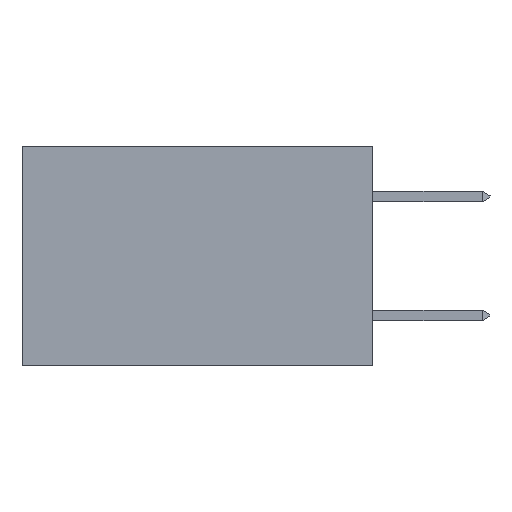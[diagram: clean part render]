
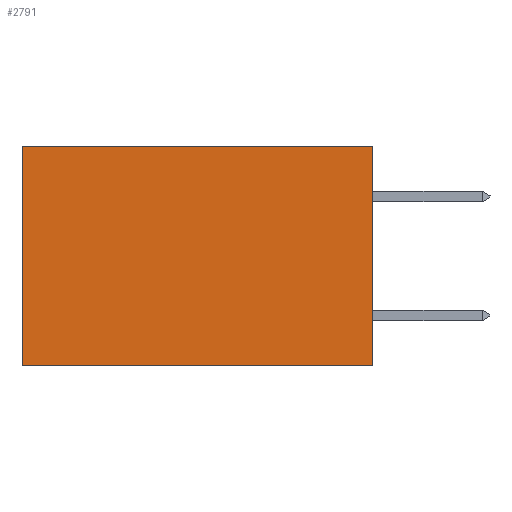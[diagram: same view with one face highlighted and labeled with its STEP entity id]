
A CAD part, left-side view. The second image highlights one B-rep face of the part: STEP entity #2791.
In plain terms, the highlighted planar face has unit normal (-1, 0, 0).
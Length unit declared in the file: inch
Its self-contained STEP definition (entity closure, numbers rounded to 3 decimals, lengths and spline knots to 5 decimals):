
#178 = VERTEX_POINT ( 'NONE', #1319 ) ;
#512 = VECTOR ( 'NONE', #5535, 39.37008 ) ;
#760 = CARTESIAN_POINT ( 'NONE',  ( 0.277, 0.59, -0.37 ) ) ;
#946 = VERTEX_POINT ( 'NONE', #2936 ) ;
#987 = VECTOR ( 'NONE', #2477, 39.37008 ) ;
#1138 = VERTEX_POINT ( 'NONE', #7677 ) ;
#1264 = EDGE_CURVE ( 'NONE', #178, #1138, #2679, .T. ) ;
#1319 = CARTESIAN_POINT ( 'NONE',  ( 0.277, 0., 0. ) ) ;
#1325 = LINE ( 'NONE', #8396, #8038 ) ;
#1663 = VECTOR ( 'NONE', #2142, 39.37008 ) ;
#1705 = DIRECTION ( 'NONE',  ( 0., 1., 0. ) ) ;
#2142 = DIRECTION ( 'NONE',  ( 0., 1., 0. ) ) ;
#2451 = EDGE_CURVE ( 'NONE', #178, #5166, #7072, .T. ) ;
#2477 = DIRECTION ( 'NONE',  ( 0., 0., -1. ) ) ;
#2679 = LINE ( 'NONE', #4357, #987 ) ;
#2791 = ADVANCED_FACE ( 'NONE', ( #5477 ), #5501, .F. ) ;
#2936 = CARTESIAN_POINT ( 'NONE',  ( 0.277, 0.59, -0.37 ) ) ;
#3075 = ORIENTED_EDGE ( 'NONE', *, *, #1264, .F. ) ;
#3343 = EDGE_LOOP ( 'NONE', ( #6837, #7013, #3075, #5827 ) ) ;
#4357 = CARTESIAN_POINT ( 'NONE',  ( 0.277, 0., -0.37 ) ) ;
#5166 = VERTEX_POINT ( 'NONE', #6594 ) ;
#5444 = EDGE_CURVE ( 'NONE', #5166, #946, #7220, .T. ) ;
#5477 = FACE_OUTER_BOUND ( 'NONE', #3343, .T. ) ;
#5501 = PLANE ( 'NONE',  #6118 ) ;
#5535 = DIRECTION ( 'NONE',  ( 0., 0., -1. ) ) ;
#5827 = ORIENTED_EDGE ( 'NONE', *, *, #2451, .T. ) ;
#5850 = EDGE_CURVE ( 'NONE', #1138, #946, #1325, .T. ) ;
#6118 = AXIS2_PLACEMENT_3D ( 'NONE', #7285, #8110, #8096 ) ;
#6594 = CARTESIAN_POINT ( 'NONE',  ( 0.277, 0.59, 0. ) ) ;
#6837 = ORIENTED_EDGE ( 'NONE', *, *, #5444, .T. ) ;
#7013 = ORIENTED_EDGE ( 'NONE', *, *, #5850, .F. ) ;
#7072 = LINE ( 'NONE', #7374, #1663 ) ;
#7220 = LINE ( 'NONE', #760, #512 ) ;
#7285 = CARTESIAN_POINT ( 'NONE',  ( 0.277, 0., -0.37 ) ) ;
#7374 = CARTESIAN_POINT ( 'NONE',  ( 0.277, 0., 0. ) ) ;
#7677 = CARTESIAN_POINT ( 'NONE',  ( 0.277, 0., -0.37 ) ) ;
#8038 = VECTOR ( 'NONE', #1705, 39.37008 ) ;
#8096 = DIRECTION ( 'NONE',  ( 0., 0., -1. ) ) ;
#8110 = DIRECTION ( 'NONE',  ( 1., 0., 0. ) ) ;
#8396 = CARTESIAN_POINT ( 'NONE',  ( 0.277, 0., -0.37 ) ) ;
